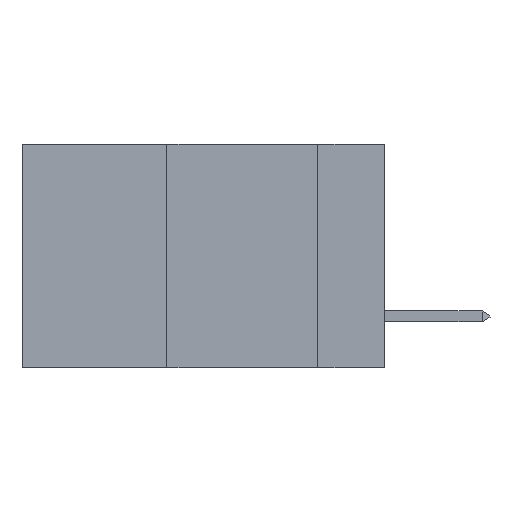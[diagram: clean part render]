
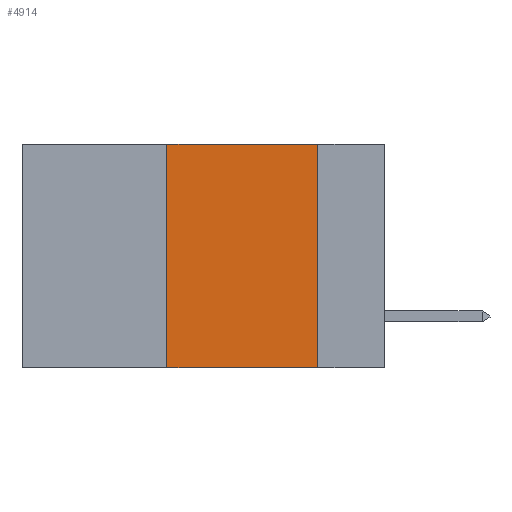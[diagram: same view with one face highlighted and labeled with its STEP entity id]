
A CAD part, left-side view. The second image highlights one B-rep face of the part: STEP entity #4914.
In plain terms, the highlighted planar face has unit normal (-1, 0, 0).
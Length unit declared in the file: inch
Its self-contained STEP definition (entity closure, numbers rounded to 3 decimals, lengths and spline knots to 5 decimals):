
#580 = LINE ( 'NONE', #10127, #3433 ) ;
#605 = EDGE_CURVE ( 'NONE', #9933, #12413, #580, .T. ) ;
#905 = CARTESIAN_POINT ( 'NONE',  ( 0., 0.36, 0. ) ) ;
#1095 = LINE ( 'NONE', #12114, #2222 ) ;
#1128 = AXIS2_PLACEMENT_3D ( 'NONE', #1421, #1376, #1360 ) ;
#1360 = DIRECTION ( 'NONE',  ( 0., 0., -1. ) ) ;
#1376 = DIRECTION ( 'NONE',  ( 1., 0., 0. ) ) ;
#1421 = CARTESIAN_POINT ( 'NONE',  ( 0., 0.6, 0. ) ) ;
#1454 = PLANE ( 'NONE',  #1128 ) ;
#2050 = ORIENTED_EDGE ( 'NONE', *, *, #4344, .F. ) ;
#2222 = VECTOR ( 'NONE', #11011, 39.37008 ) ;
#3098 = CARTESIAN_POINT ( 'NONE',  ( 0., 0.6, 0. ) ) ;
#3156 = LINE ( 'NONE', #3098, #15121 ) ;
#3293 = EDGE_LOOP ( 'NONE', ( #5326, #2050, #4072, #7040 ) ) ;
#3433 = VECTOR ( 'NONE', #10215, 39.37008 ) ;
#3814 = CARTESIAN_POINT ( 'NONE',  ( 0., 0.11, 0. ) ) ;
#4072 = ORIENTED_EDGE ( 'NONE', *, *, #11968, .F. ) ;
#4344 = EDGE_CURVE ( 'NONE', #6703, #13256, #3156, .T. ) ;
#4372 = DIRECTION ( 'NONE',  ( 0., -1., 0. ) ) ;
#4914 = ADVANCED_FACE ( 'NONE', ( #14456 ), #1454, .F. ) ;
#4924 = CARTESIAN_POINT ( 'NONE',  ( 0., 0.36, -0.37 ) ) ;
#5055 = DIRECTION ( 'NONE',  ( 0., 0., -1. ) ) ;
#5326 = ORIENTED_EDGE ( 'NONE', *, *, #9334, .F. ) ;
#6237 = VECTOR ( 'NONE', #5055, 39.37008 ) ;
#6703 = VERTEX_POINT ( 'NONE', #905 ) ;
#7040 = ORIENTED_EDGE ( 'NONE', *, *, #605, .T. ) ;
#7748 = CARTESIAN_POINT ( 'NONE',  ( 0., 0.11, -0.37 ) ) ;
#9334 = EDGE_CURVE ( 'NONE', #13256, #12413, #9418, .T. ) ;
#9418 = LINE ( 'NONE', #3814, #6237 ) ;
#9933 = VERTEX_POINT ( 'NONE', #4924 ) ;
#10127 = CARTESIAN_POINT ( 'NONE',  ( 0., 0.6, -0.37 ) ) ;
#10215 = DIRECTION ( 'NONE',  ( 0., -1., 0. ) ) ;
#11011 = DIRECTION ( 'NONE',  ( 0., 0., 1. ) ) ;
#11968 = EDGE_CURVE ( 'NONE', #9933, #6703, #1095, .T. ) ;
#12114 = CARTESIAN_POINT ( 'NONE',  ( 0., 0.36, 0. ) ) ;
#12125 = CARTESIAN_POINT ( 'NONE',  ( 0., 0.11, 0. ) ) ;
#12413 = VERTEX_POINT ( 'NONE', #7748 ) ;
#13256 = VERTEX_POINT ( 'NONE', #12125 ) ;
#14456 = FACE_OUTER_BOUND ( 'NONE', #3293, .T. ) ;
#15121 = VECTOR ( 'NONE', #4372, 39.37008 ) ;
